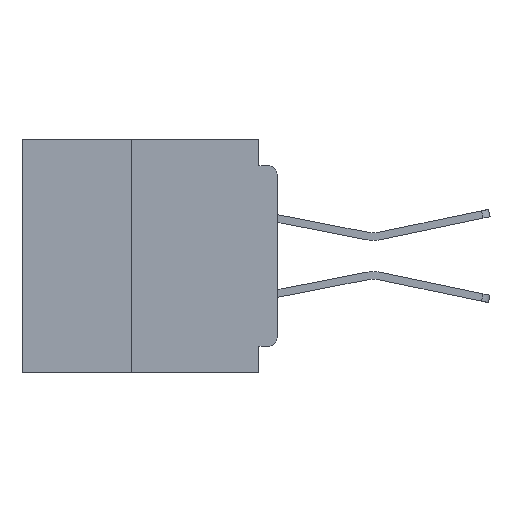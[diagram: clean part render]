
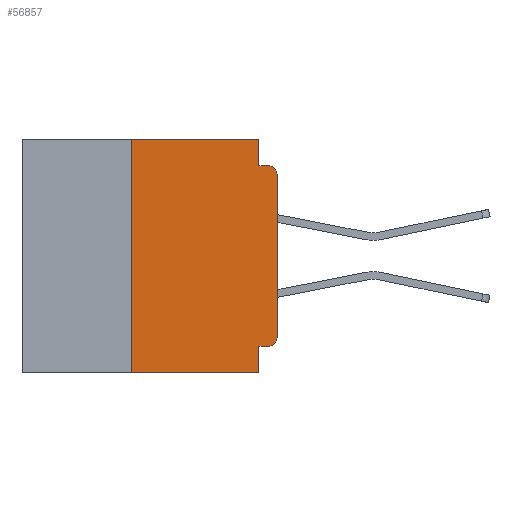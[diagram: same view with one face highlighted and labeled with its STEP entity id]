
A CAD part, left-side view. The second image highlights one B-rep face of the part: STEP entity #56857.
In plain terms, the highlighted planar face has unit normal (-1, 0, 0).
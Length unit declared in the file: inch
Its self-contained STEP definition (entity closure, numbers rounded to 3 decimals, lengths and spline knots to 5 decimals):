
#53 = VERTEX_POINT ( 'NONE', #53731 ) ;
#400 = VECTOR ( 'NONE', #26731, 39.37008 ) ;
#1214 = VERTEX_POINT ( 'NONE', #54944 ) ;
#1972 = DIRECTION ( 'NONE',  ( 0., 0., -1. ) ) ;
#2515 = VECTOR ( 'NONE', #24562, 39.37008 ) ;
#3193 = VERTEX_POINT ( 'NONE', #42642 ) ;
#4632 = ORIENTED_EDGE ( 'NONE', *, *, #16933, .T. ) ;
#4754 = AXIS2_PLACEMENT_3D ( 'NONE', #56422, #29203, #1972 ) ;
#7621 = DIRECTION ( 'NONE',  ( -1., 0., 0. ) ) ;
#8967 = EDGE_CURVE ( 'NONE', #1214, #11112, #19185, .T. ) ;
#9320 = CARTESIAN_POINT ( 'NONE',  ( 0., 0.437, 0. ) ) ;
#10732 = LINE ( 'NONE', #43875, #37735 ) ;
#11104 = ORIENTED_EDGE ( 'NONE', *, *, #37042, .F. ) ;
#11112 = VERTEX_POINT ( 'NONE', #37049 ) ;
#11220 = VERTEX_POINT ( 'NONE', #56116 ) ;
#11630 = FACE_OUTER_BOUND ( 'NONE', #53014, .T. ) ;
#11833 = CARTESIAN_POINT ( 'NONE',  ( 0., 0.031, -0.045 ) ) ;
#12532 = LINE ( 'NONE', #22132, #400 ) ;
#13829 = CARTESIAN_POINT ( 'NONE',  ( 0., 0., -0.355 ) ) ;
#13872 = DIRECTION ( 'NONE',  ( 0., -1., 0. ) ) ;
#14968 = PLANE ( 'NONE',  #47680 ) ;
#15453 = EDGE_CURVE ( 'NONE', #22957, #3193, #36250, .T. ) ;
#15840 = CARTESIAN_POINT ( 'NONE',  ( 0., 0., 0. ) ) ;
#15881 = CARTESIAN_POINT ( 'NONE',  ( 0., 0., -0.34 ) ) ;
#16933 = EDGE_CURVE ( 'NONE', #46693, #1214, #28951, .T. ) ;
#17740 = ORIENTED_EDGE ( 'NONE', *, *, #49666, .T. ) ;
#19185 = CIRCLE ( 'NONE', #50550, 0.015 ) ;
#19483 = CARTESIAN_POINT ( 'NONE',  ( 0., 0.437, 0. ) ) ;
#19557 = ORIENTED_EDGE ( 'NONE', *, *, #58382, .F. ) ;
#20099 = ORIENTED_EDGE ( 'NONE', *, *, #43204, .T. ) ;
#22132 = CARTESIAN_POINT ( 'NONE',  ( 0., 0.25, -0.4 ) ) ;
#22855 = LINE ( 'NONE', #13829, #57745 ) ;
#22957 = VERTEX_POINT ( 'NONE', #23235 ) ;
#23235 = CARTESIAN_POINT ( 'NONE',  ( 0., 0.25, 0. ) ) ;
#23333 = ORIENTED_EDGE ( 'NONE', *, *, #24136, .F. ) ;
#24076 = DIRECTION ( 'NONE',  ( 1., 0., 0. ) ) ;
#24136 = EDGE_CURVE ( 'NONE', #53, #28459, #22855, .T. ) ;
#24562 = DIRECTION ( 'NONE',  ( 0., -1., 0. ) ) ;
#24998 = DIRECTION ( 'NONE',  ( 0., 0., 1. ) ) ;
#26679 = LINE ( 'NONE', #51796, #2515 ) ;
#26731 = DIRECTION ( 'NONE',  ( 0., 0., 1. ) ) ;
#27320 = VERTEX_POINT ( 'NONE', #11833 ) ;
#27519 = VECTOR ( 'NONE', #24998, 39.37008 ) ;
#27868 = VECTOR ( 'NONE', #54775, 39.37008 ) ;
#28329 = VERTEX_POINT ( 'NONE', #49158 ) ;
#28459 = VERTEX_POINT ( 'NONE', #31810 ) ;
#28951 = LINE ( 'NONE', #15840, #27519 ) ;
#29203 = DIRECTION ( 'NONE',  ( -1., 0., 0. ) ) ;
#30104 = CARTESIAN_POINT ( 'NONE',  ( 0., 0.031, -0.4 ) ) ;
#31810 = CARTESIAN_POINT ( 'NONE',  ( 0., 0.031, -0.355 ) ) ;
#34774 = CARTESIAN_POINT ( 'NONE',  ( 0., 0.015, -0.06 ) ) ;
#34829 = VECTOR ( 'NONE', #13872, 39.37008 ) ;
#34868 = DIRECTION ( 'NONE',  ( 0., 0., -1. ) ) ;
#36250 = LINE ( 'NONE', #9320, #34829 ) ;
#36305 = CARTESIAN_POINT ( 'NONE',  ( 0., 0., -0.045 ) ) ;
#37042 = EDGE_CURVE ( 'NONE', #28459, #11220, #55323, .T. ) ;
#37049 = CARTESIAN_POINT ( 'NONE',  ( 0., 0.015, -0.045 ) ) ;
#37735 = VECTOR ( 'NONE', #57540, 39.37008 ) ;
#39395 = DIRECTION ( 'NONE',  ( 0., 0., -1. ) ) ;
#39994 = LINE ( 'NONE', #36305, #27868 ) ;
#40424 = VECTOR ( 'NONE', #34868, 39.37008 ) ;
#42642 = CARTESIAN_POINT ( 'NONE',  ( 0., 0.031, 0. ) ) ;
#43204 = EDGE_CURVE ( 'NONE', #28329, #11220, #26679, .T. ) ;
#43875 = CARTESIAN_POINT ( 'NONE',  ( 0., 0.031, 0. ) ) ;
#43984 = ORIENTED_EDGE ( 'NONE', *, *, #51552, .F. ) ;
#46693 = VERTEX_POINT ( 'NONE', #15881 ) ;
#47680 = AXIS2_PLACEMENT_3D ( 'NONE', #19483, #24076, #55893 ) ;
#49158 = CARTESIAN_POINT ( 'NONE',  ( 0., 0.25, -0.4 ) ) ;
#49666 = EDGE_CURVE ( 'NONE', #53, #46693, #58592, .T. ) ;
#50550 = AXIS2_PLACEMENT_3D ( 'NONE', #34774, #7621, #39395 ) ;
#51552 = EDGE_CURVE ( 'NONE', #27320, #11112, #39994, .T. ) ;
#51796 = CARTESIAN_POINT ( 'NONE',  ( 0., 0.437, -0.4 ) ) ;
#52589 = ORIENTED_EDGE ( 'NONE', *, *, #15453, .F. ) ;
#53014 = EDGE_LOOP ( 'NONE', ( #4632, #55657, #43984, #19557, #52589, #56202, #20099, #11104, #23333, #17740 ) ) ;
#53731 = CARTESIAN_POINT ( 'NONE',  ( 0., 0.015, -0.355 ) ) ;
#54537 = DIRECTION ( 'NONE',  ( 0., 1., 0. ) ) ;
#54775 = DIRECTION ( 'NONE',  ( 0., -1., 0. ) ) ;
#54944 = CARTESIAN_POINT ( 'NONE',  ( 0., 0., -0.06 ) ) ;
#55313 = EDGE_CURVE ( 'NONE', #28329, #22957, #12532, .T. ) ;
#55323 = LINE ( 'NONE', #30104, #40424 ) ;
#55657 = ORIENTED_EDGE ( 'NONE', *, *, #8967, .T. ) ;
#55893 = DIRECTION ( 'NONE',  ( 0., 0., -1. ) ) ;
#56116 = CARTESIAN_POINT ( 'NONE',  ( 0., 0.031, -0.4 ) ) ;
#56202 = ORIENTED_EDGE ( 'NONE', *, *, #55313, .F. ) ;
#56422 = CARTESIAN_POINT ( 'NONE',  ( 0., 0.015, -0.34 ) ) ;
#56857 = ADVANCED_FACE ( 'NONE', ( #11630 ), #14968, .F. ) ;
#57540 = DIRECTION ( 'NONE',  ( 0., 0., -1. ) ) ;
#57745 = VECTOR ( 'NONE', #54537, 39.37008 ) ;
#58382 = EDGE_CURVE ( 'NONE', #3193, #27320, #10732, .T. ) ;
#58592 = CIRCLE ( 'NONE', #4754, 0.015 ) ;
